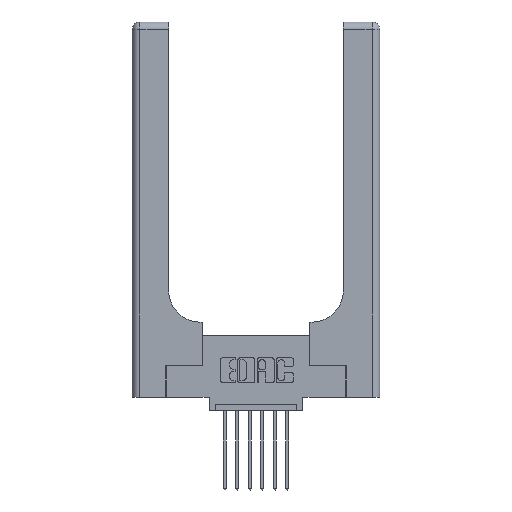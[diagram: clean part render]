
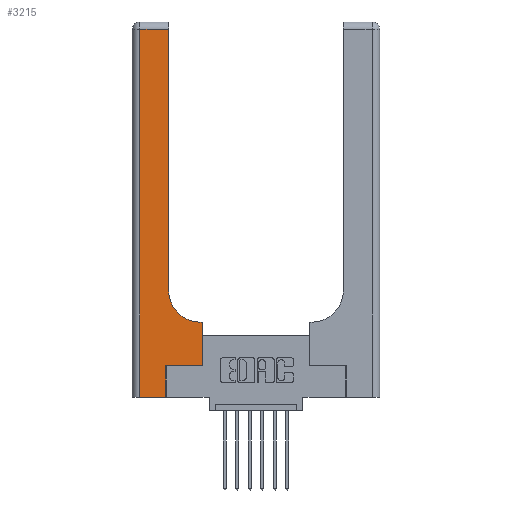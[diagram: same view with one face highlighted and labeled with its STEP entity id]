
A CAD part, top view. The second image highlights one B-rep face of the part: STEP entity #3215.
In plain terms, the highlighted planar face has unit normal (0, 0, 1).
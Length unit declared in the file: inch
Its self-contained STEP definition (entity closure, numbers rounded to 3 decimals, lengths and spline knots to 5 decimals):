
#115 = DIRECTION ( 'NONE',  ( -1., 0., 0. ) ) ;
#434 = LINE ( 'NONE', #13313, #1166 ) ;
#766 = LINE ( 'NONE', #11805, #1814 ) ;
#1166 = VECTOR ( 'NONE', #3024, 39.37008 ) ;
#1308 = CARTESIAN_POINT ( 'NONE',  ( 0., 2.94, 0.37 ) ) ;
#1415 = EDGE_CURVE ( 'NONE', #13100, #9386, #4532, .T. ) ;
#1470 = VERTEX_POINT ( 'NONE', #7082 ) ;
#1654 = ORIENTED_EDGE ( 'NONE', *, *, #10545, .T. ) ;
#1730 = AXIS2_PLACEMENT_3D ( 'NONE', #1743, #13012, #10782 ) ;
#1743 = CARTESIAN_POINT ( 'NONE',  ( 0.5415, 0.85, 0.37 ) ) ;
#1757 = CARTESIAN_POINT ( 'NONE',  ( 0.2915, 3., 0.37 ) ) ;
#1806 = DIRECTION ( 'NONE',  ( 0., 0., -1. ) ) ;
#1814 = VECTOR ( 'NONE', #12940, 39.37008 ) ;
#1830 = ORIENTED_EDGE ( 'NONE', *, *, #7244, .T. ) ;
#1866 = CARTESIAN_POINT ( 'NONE',  ( 0.2915, 0.85, 0.37 ) ) ;
#2010 = CARTESIAN_POINT ( 'NONE',  ( 0.269, 0.25, 0.37 ) ) ;
#2273 = VERTEX_POINT ( 'NONE', #1866 ) ;
#2717 = VECTOR ( 'NONE', #12959, 39.37008 ) ;
#3024 = DIRECTION ( 'NONE',  ( -1., 0., 0. ) ) ;
#3215 = ADVANCED_FACE ( 'NONE', ( #5387 ), #10951, .F. ) ;
#4016 = ORIENTED_EDGE ( 'NONE', *, *, #5306, .T. ) ;
#4051 = EDGE_LOOP ( 'NONE', ( #1830, #8674, #11920, #1654, #7428, #4016, #5532, #8499, #5844 ) ) ;
#4138 = DIRECTION ( 'NONE',  ( -1., 0., 0. ) ) ;
#4457 = CARTESIAN_POINT ( 'NONE',  ( 0.06, 2.94, 0.37 ) ) ;
#4532 = LINE ( 'NONE', #1308, #7015 ) ;
#5115 = EDGE_CURVE ( 'NONE', #9386, #12432, #766, .T. ) ;
#5247 = EDGE_CURVE ( 'NONE', #1470, #10184, #8730, .T. ) ;
#5306 = EDGE_CURVE ( 'NONE', #10184, #11577, #8714, .T. ) ;
#5326 = DIRECTION ( 'NONE',  ( 1., 0., 0. ) ) ;
#5387 = FACE_OUTER_BOUND ( 'NONE', #4051, .T. ) ;
#5532 = ORIENTED_EDGE ( 'NONE', *, *, #10194, .T. ) ;
#5660 = VERTEX_POINT ( 'NONE', #14353 ) ;
#5844 = ORIENTED_EDGE ( 'NONE', *, *, #7908, .T. ) ;
#6134 = DIRECTION ( 'NONE',  ( 0., 1., 0. ) ) ;
#6446 = LINE ( 'NONE', #10898, #13239 ) ;
#7015 = VECTOR ( 'NONE', #115, 39.37008 ) ;
#7082 = CARTESIAN_POINT ( 'NONE',  ( 0.269, 0., 0.37 ) ) ;
#7181 = CARTESIAN_POINT ( 'NONE',  ( 0.269, 0., 0.37 ) ) ;
#7198 = CARTESIAN_POINT ( 'NONE',  ( 0.5585, 0.25, 0.37 ) ) ;
#7244 = EDGE_CURVE ( 'NONE', #2273, #13100, #10814, .T. ) ;
#7428 = ORIENTED_EDGE ( 'NONE', *, *, #5247, .T. ) ;
#7705 = CARTESIAN_POINT ( 'NONE',  ( 0.2915, 2.94, 0.37 ) ) ;
#7908 = EDGE_CURVE ( 'NONE', #12669, #2273, #11693, .T. ) ;
#8215 = LINE ( 'NONE', #12911, #13756 ) ;
#8499 = ORIENTED_EDGE ( 'NONE', *, *, #10806, .T. ) ;
#8674 = ORIENTED_EDGE ( 'NONE', *, *, #1415, .T. ) ;
#8714 = LINE ( 'NONE', #2010, #13886 ) ;
#8730 = LINE ( 'NONE', #7181, #2717 ) ;
#9386 = VERTEX_POINT ( 'NONE', #4457 ) ;
#9413 = CARTESIAN_POINT ( 'NONE',  ( 0.5415, 0.6, 0.37 ) ) ;
#9610 = CARTESIAN_POINT ( 'NONE',  ( 0.06, 0., 0.37 ) ) ;
#10184 = VERTEX_POINT ( 'NONE', #13229 ) ;
#10194 = EDGE_CURVE ( 'NONE', #11577, #5660, #6446, .T. ) ;
#10545 = EDGE_CURVE ( 'NONE', #12432, #1470, #8215, .T. ) ;
#10782 = DIRECTION ( 'NONE',  ( 1., 0., 0. ) ) ;
#10806 = EDGE_CURVE ( 'NONE', #5660, #12669, #434, .T. ) ;
#10814 = LINE ( 'NONE', #1757, #12945 ) ;
#10898 = CARTESIAN_POINT ( 'NONE',  ( 0.5585, 0.25, 0.37 ) ) ;
#10951 = PLANE ( 'NONE',  #14715 ) ;
#11577 = VERTEX_POINT ( 'NONE', #7198 ) ;
#11693 = CIRCLE ( 'NONE', #1730, 0.25 ) ;
#11805 = CARTESIAN_POINT ( 'NONE',  ( 0.06, 3., 0.37 ) ) ;
#11920 = ORIENTED_EDGE ( 'NONE', *, *, #5115, .T. ) ;
#12432 = VERTEX_POINT ( 'NONE', #9610 ) ;
#12669 = VERTEX_POINT ( 'NONE', #9413 ) ;
#12911 = CARTESIAN_POINT ( 'NONE',  ( 0., 0., 0.37 ) ) ;
#12940 = DIRECTION ( 'NONE',  ( 0., -1., 0. ) ) ;
#12945 = VECTOR ( 'NONE', #6134, 39.37008 ) ;
#12959 = DIRECTION ( 'NONE',  ( 0., 1., 0. ) ) ;
#13012 = DIRECTION ( 'NONE',  ( 0., 0., -1. ) ) ;
#13100 = VERTEX_POINT ( 'NONE', #7705 ) ;
#13229 = CARTESIAN_POINT ( 'NONE',  ( 0.269, 0.25, 0.37 ) ) ;
#13239 = VECTOR ( 'NONE', #14413, 39.37008 ) ;
#13313 = CARTESIAN_POINT ( 'NONE',  ( 0.2915, 0.6, 0.37 ) ) ;
#13756 = VECTOR ( 'NONE', #13908, 39.37008 ) ;
#13886 = VECTOR ( 'NONE', #5326, 39.37008 ) ;
#13908 = DIRECTION ( 'NONE',  ( 1., 0., 0. ) ) ;
#14209 = CARTESIAN_POINT ( 'NONE',  ( 0., 3., 0.37 ) ) ;
#14353 = CARTESIAN_POINT ( 'NONE',  ( 0.5585, 0.6, 0.37 ) ) ;
#14413 = DIRECTION ( 'NONE',  ( 0., 1., 0. ) ) ;
#14715 = AXIS2_PLACEMENT_3D ( 'NONE', #14209, #1806, #4138 ) ;
